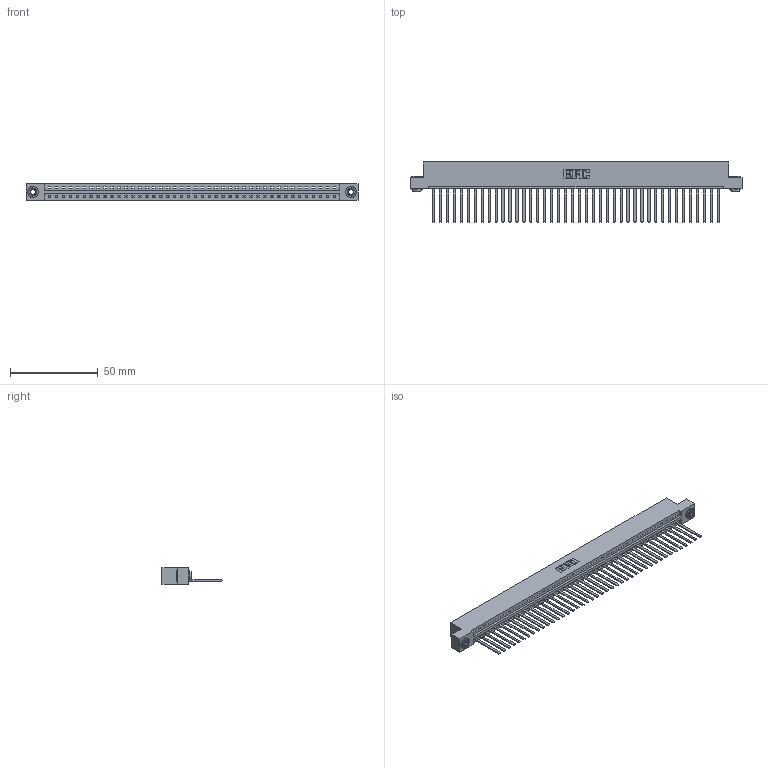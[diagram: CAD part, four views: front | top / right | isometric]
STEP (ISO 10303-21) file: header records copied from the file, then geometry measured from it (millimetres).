
FILE_DESCRIPTION (( 'STEP AP203' ), '1' );
FILE_NAME ('387-042-544-103.STEP', '2018-09-19T23:05:30', ( '' ), ( '' ), 'SwSTEP 2.0', 'SolidWorks 2016', '' );
FILE_SCHEMA (( 'CONFIG_CONTROL_DESIGN' ));
Length unit declared in the file: inch
Products named in the file (4): 387-042-544-103; 337 Part_Flush Mounting Lugs - 0.156 Dia-TH; 345-292-001_345-293-144; 345-250-002_345-250-002-102
Assembly tree (45 placements, depth 2):
  387-042-544-103
    337 Part_Flush Mounting Lugs - 0.156 Dia-TH
    345-292-001_345-293-144  x42
    345-250-002_345-250-002-102  x2
Bounding box: 189.43 x 34.3 x 9.4 mm (x, y, z)
Volume: 20194.2 mm3; surface area: 22700.5 mm2
Topology: 45 solids, 45 shells, 2504 faces, 7527 edges, 4958 vertices
Faces by surface type: plane 1844, cylinder 652, cone 8
Entity records: 31686 total; most frequent: CARTESIAN_POINT 5495, ORIENTED_EDGE 5466, DIRECTION 4655, EDGE_CURVE 2733, VECTOR 2585, LINE 2585, VERTEX_POINT 1818, AXIS2_PLACEMENT_3D 1035
